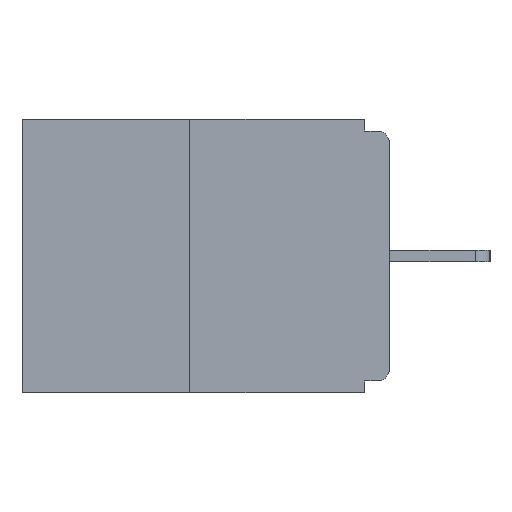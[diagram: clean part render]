
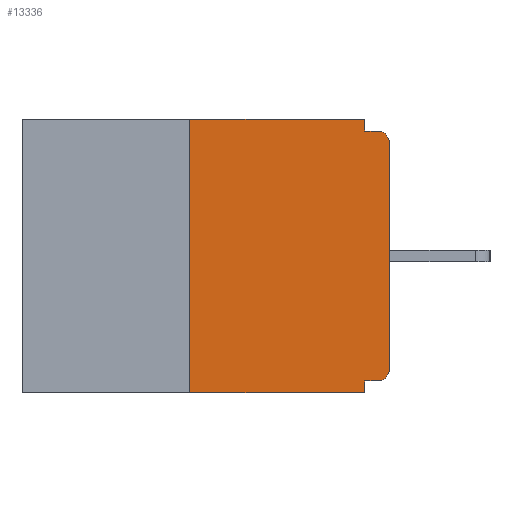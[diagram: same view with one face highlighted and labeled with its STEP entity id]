
A CAD part, left-side view. The second image highlights one B-rep face of the part: STEP entity #13336.
In plain terms, the highlighted planar face has unit normal (-1, 0, 0).
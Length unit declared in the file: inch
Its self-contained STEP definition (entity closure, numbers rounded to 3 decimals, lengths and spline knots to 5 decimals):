
#32 = VERTEX_POINT ( 'NONE', #18467 ) ;
#48 = ORIENTED_EDGE ( 'NONE', *, *, #7293, .T. ) ;
#100 = CARTESIAN_POINT ( 'NONE',  ( 0., 0.015, -0.313 ) ) ;
#164 = VECTOR ( 'NONE', #8927, 39.37008 ) ;
#326 = VECTOR ( 'NONE', #6073, 39.37008 ) ;
#1603 = CARTESIAN_POINT ( 'NONE',  ( 0., 0.015, -0.03 ) ) ;
#1800 = ORIENTED_EDGE ( 'NONE', *, *, #7139, .F. ) ;
#1818 = CARTESIAN_POINT ( 'NONE',  ( 0., 0.031, 0. ) ) ;
#2887 = CARTESIAN_POINT ( 'NONE',  ( 0., 0.031, -0.015 ) ) ;
#2890 = VERTEX_POINT ( 'NONE', #18606 ) ;
#2930 = DIRECTION ( 'NONE',  ( 0., 0., -1. ) ) ;
#2963 = VECTOR ( 'NONE', #2930, 39.37008 ) ;
#3474 = CARTESIAN_POINT ( 'NONE',  ( 0., 0.25, 0. ) ) ;
#3628 = ORIENTED_EDGE ( 'NONE', *, *, #21042, .F. ) ;
#3896 = PLANE ( 'NONE',  #6864 ) ;
#4137 = AXIS2_PLACEMENT_3D ( 'NONE', #1603, #11268, #14744 ) ;
#4897 = DIRECTION ( 'NONE',  ( 0., 0., 1. ) ) ;
#5151 = LINE ( 'NONE', #20673, #326 ) ;
#5708 = CARTESIAN_POINT ( 'NONE',  ( 0., 0.031, 0. ) ) ;
#6073 = DIRECTION ( 'NONE',  ( 0., -1., 0. ) ) ;
#6076 = LINE ( 'NONE', #17868, #20562 ) ;
#6107 = DIRECTION ( 'NONE',  ( 0., 0., 1. ) ) ;
#6379 = EDGE_CURVE ( 'NONE', #32, #12621, #16304, .T. ) ;
#6695 = AXIS2_PLACEMENT_3D ( 'NONE', #100, #18158, #19779 ) ;
#6762 = EDGE_CURVE ( 'NONE', #12200, #6777, #6076, .T. ) ;
#6777 = VERTEX_POINT ( 'NONE', #3474 ) ;
#6864 = AXIS2_PLACEMENT_3D ( 'NONE', #15290, #13777, #20034 ) ;
#6870 = VECTOR ( 'NONE', #15773, 39.37008 ) ;
#7009 = VERTEX_POINT ( 'NONE', #11264 ) ;
#7139 = EDGE_CURVE ( 'NONE', #10419, #15114, #21007, .T. ) ;
#7293 = EDGE_CURVE ( 'NONE', #7009, #32, #11166, .T. ) ;
#7298 = EDGE_LOOP ( 'NONE', ( #20187, #15695, #16213, #11608, #3628, #48, #8392, #12333, #8252, #1800 ) ) ;
#7506 = CARTESIAN_POINT ( 'NONE',  ( 0., 0.46, -0.343 ) ) ;
#7520 = DIRECTION ( 'NONE',  ( 0., 1., 0. ) ) ;
#8013 = LINE ( 'NONE', #17280, #19191 ) ;
#8252 = ORIENTED_EDGE ( 'NONE', *, *, #16352, .F. ) ;
#8392 = ORIENTED_EDGE ( 'NONE', *, *, #6379, .T. ) ;
#8583 = EDGE_CURVE ( 'NONE', #6777, #10419, #14039, .T. ) ;
#8927 = DIRECTION ( 'NONE',  ( 0., 0., -1. ) ) ;
#9706 = VECTOR ( 'NONE', #12237, 39.37008 ) ;
#10400 = CARTESIAN_POINT ( 'NONE',  ( 0., 0.46, 0. ) ) ;
#10419 = VERTEX_POINT ( 'NONE', #1818 ) ;
#10727 = LINE ( 'NONE', #7506, #6870 ) ;
#11166 = CIRCLE ( 'NONE', #6695, 0.015 ) ;
#11264 = CARTESIAN_POINT ( 'NONE',  ( 0., 0.015, -0.328 ) ) ;
#11268 = DIRECTION ( 'NONE',  ( -1., 0., 0. ) ) ;
#11608 = ORIENTED_EDGE ( 'NONE', *, *, #20432, .F. ) ;
#12200 = VERTEX_POINT ( 'NONE', #13956 ) ;
#12237 = DIRECTION ( 'NONE',  ( 0., -1., 0. ) ) ;
#12333 = ORIENTED_EDGE ( 'NONE', *, *, #13559, .T. ) ;
#12413 = CARTESIAN_POINT ( 'NONE',  ( 0., 0.031, -0.343 ) ) ;
#12621 = VERTEX_POINT ( 'NONE', #16402 ) ;
#13336 = ADVANCED_FACE ( 'NONE', ( #15212 ), #3896, .F. ) ;
#13559 = EDGE_CURVE ( 'NONE', #12621, #14832, #18755, .T. ) ;
#13777 = DIRECTION ( 'NONE',  ( 1., 0., 0. ) ) ;
#13956 = CARTESIAN_POINT ( 'NONE',  ( 0., 0.25, -0.343 ) ) ;
#14039 = LINE ( 'NONE', #10400, #9706 ) ;
#14280 = VECTOR ( 'NONE', #6107, 39.37008 ) ;
#14567 = CARTESIAN_POINT ( 'NONE',  ( 0., 0.031, -0.343 ) ) ;
#14635 = VERTEX_POINT ( 'NONE', #14567 ) ;
#14744 = DIRECTION ( 'NONE',  ( 0., 0., -1. ) ) ;
#14832 = VERTEX_POINT ( 'NONE', #17885 ) ;
#15114 = VERTEX_POINT ( 'NONE', #2887 ) ;
#15212 = FACE_OUTER_BOUND ( 'NONE', #7298, .T. ) ;
#15290 = CARTESIAN_POINT ( 'NONE',  ( 0., 0.46, 0. ) ) ;
#15419 = LINE ( 'NONE', #12413, #164 ) ;
#15695 = ORIENTED_EDGE ( 'NONE', *, *, #6762, .F. ) ;
#15773 = DIRECTION ( 'NONE',  ( 0., -1., 0. ) ) ;
#16213 = ORIENTED_EDGE ( 'NONE', *, *, #17643, .T. ) ;
#16304 = LINE ( 'NONE', #17421, #14280 ) ;
#16352 = EDGE_CURVE ( 'NONE', #15114, #14832, #5151, .T. ) ;
#16402 = CARTESIAN_POINT ( 'NONE',  ( 0., 0., -0.03 ) ) ;
#17280 = CARTESIAN_POINT ( 'NONE',  ( 0., 0., -0.328 ) ) ;
#17421 = CARTESIAN_POINT ( 'NONE',  ( 0., 0., 0. ) ) ;
#17643 = EDGE_CURVE ( 'NONE', #12200, #14635, #10727, .T. ) ;
#17868 = CARTESIAN_POINT ( 'NONE',  ( 0., 0.25, 0. ) ) ;
#17885 = CARTESIAN_POINT ( 'NONE',  ( 0., 0.015, -0.015 ) ) ;
#18158 = DIRECTION ( 'NONE',  ( -1., 0., 0. ) ) ;
#18467 = CARTESIAN_POINT ( 'NONE',  ( 0., 0., -0.313 ) ) ;
#18606 = CARTESIAN_POINT ( 'NONE',  ( 0., 0.031, -0.328 ) ) ;
#18755 = CIRCLE ( 'NONE', #4137, 0.015 ) ;
#19191 = VECTOR ( 'NONE', #7520, 39.37008 ) ;
#19779 = DIRECTION ( 'NONE',  ( 0., 0., -1. ) ) ;
#20034 = DIRECTION ( 'NONE',  ( 0., 0., -1. ) ) ;
#20187 = ORIENTED_EDGE ( 'NONE', *, *, #8583, .F. ) ;
#20432 = EDGE_CURVE ( 'NONE', #2890, #14635, #15419, .T. ) ;
#20562 = VECTOR ( 'NONE', #4897, 39.37008 ) ;
#20673 = CARTESIAN_POINT ( 'NONE',  ( 0., 0., -0.015 ) ) ;
#21007 = LINE ( 'NONE', #5708, #2963 ) ;
#21042 = EDGE_CURVE ( 'NONE', #7009, #2890, #8013, .T. ) ;
